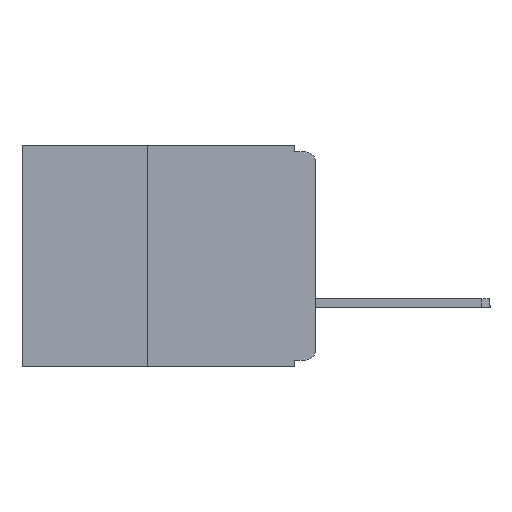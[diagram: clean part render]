
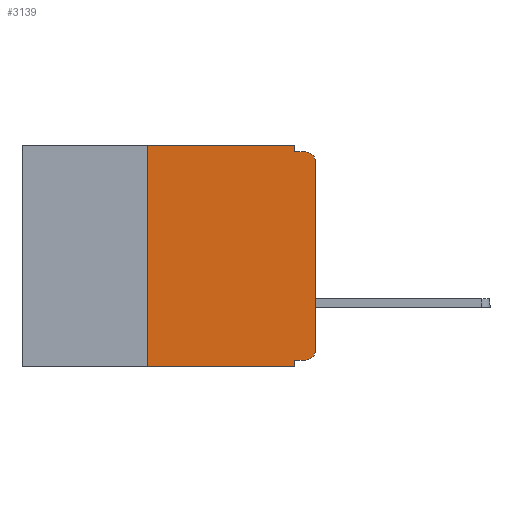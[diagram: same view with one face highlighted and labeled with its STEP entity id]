
A CAD part, left-side view. The second image highlights one B-rep face of the part: STEP entity #3139.
In plain terms, the highlighted planar face has unit normal (-1, 0, 0).
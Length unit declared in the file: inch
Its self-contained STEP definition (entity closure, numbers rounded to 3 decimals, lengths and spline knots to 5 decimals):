
#608 = LINE ( 'NONE', #33275, #14119 ) ;
#1898 = CARTESIAN_POINT ( 'NONE',  ( 0., 0.25, -0.33 ) ) ;
#2515 = CARTESIAN_POINT ( 'NONE',  ( 0., 0., 0. ) ) ;
#2566 = CARTESIAN_POINT ( 'NONE',  ( 0., 0.25, 0. ) ) ;
#3139 = ADVANCED_FACE ( 'NONE', ( #21824 ), #23279, .F. ) ;
#3199 = VERTEX_POINT ( 'NONE', #20405 ) ;
#3339 = ORIENTED_EDGE ( 'NONE', *, *, #6237, .F. ) ;
#4560 = LINE ( 'NONE', #33497, #31786 ) ;
#4748 = VERTEX_POINT ( 'NONE', #15041 ) ;
#5008 = CARTESIAN_POINT ( 'NONE',  ( 0., 0.015, -0.01 ) ) ;
#5044 = ORIENTED_EDGE ( 'NONE', *, *, #23647, .F. ) ;
#5058 = EDGE_LOOP ( 'NONE', ( #14298, #30668, #3339, #17620, #5044, #19236, #20870, #14730, #24922, #26579 ) ) ;
#5066 = VERTEX_POINT ( 'NONE', #10063 ) ;
#5344 = VERTEX_POINT ( 'NONE', #5008 ) ;
#5738 = VECTOR ( 'NONE', #20598, 39.37008 ) ;
#6003 = DIRECTION ( 'NONE',  ( -1., 0., 0. ) ) ;
#6237 = EDGE_CURVE ( 'NONE', #25478, #5344, #15923, .T. ) ;
#6511 = VERTEX_POINT ( 'NONE', #30363 ) ;
#6776 = VERTEX_POINT ( 'NONE', #28749 ) ;
#7833 = EDGE_CURVE ( 'NONE', #6776, #23293, #20725, .T. ) ;
#7985 = VECTOR ( 'NONE', #23960, 39.37008 ) ;
#8428 = EDGE_CURVE ( 'NONE', #5066, #16744, #608, .T. ) ;
#8774 = LINE ( 'NONE', #23782, #21980 ) ;
#8851 = LINE ( 'NONE', #25400, #15092 ) ;
#10063 = CARTESIAN_POINT ( 'NONE',  ( 0., 0.031, -0.32 ) ) ;
#10379 = VERTEX_POINT ( 'NONE', #13954 ) ;
#11586 = AXIS2_PLACEMENT_3D ( 'NONE', #22886, #22854, #22810 ) ;
#12396 = DIRECTION ( 'NONE',  ( 0., 0., -1. ) ) ;
#12749 = DIRECTION ( 'NONE',  ( 0., 1., 0. ) ) ;
#13954 = CARTESIAN_POINT ( 'NONE',  ( 0., 0.015, -0.32 ) ) ;
#14119 = VECTOR ( 'NONE', #12396, 39.37008 ) ;
#14218 = AXIS2_PLACEMENT_3D ( 'NONE', #21885, #6003, #24488 ) ;
#14298 = ORIENTED_EDGE ( 'NONE', *, *, #17887, .T. ) ;
#14347 = CARTESIAN_POINT ( 'NONE',  ( 0., 0.015, -0.305 ) ) ;
#14730 = ORIENTED_EDGE ( 'NONE', *, *, #8428, .F. ) ;
#15041 = CARTESIAN_POINT ( 'NONE',  ( 0., 0., -0.025 ) ) ;
#15092 = VECTOR ( 'NONE', #28047, 39.37008 ) ;
#15923 = LINE ( 'NONE', #21362, #7985 ) ;
#16331 = EDGE_CURVE ( 'NONE', #10379, #5066, #4560, .T. ) ;
#16744 = VERTEX_POINT ( 'NONE', #22338 ) ;
#16999 = DIRECTION ( 'NONE',  ( 0., 0., -1. ) ) ;
#17432 = VECTOR ( 'NONE', #18570, 39.37008 ) ;
#17620 = ORIENTED_EDGE ( 'NONE', *, *, #28528, .F. ) ;
#17887 = EDGE_CURVE ( 'NONE', #3199, #4748, #23500, .T. ) ;
#18570 = DIRECTION ( 'NONE',  ( 0., 0., 1. ) ) ;
#18691 = DIRECTION ( 'NONE',  ( 0., -1., 0. ) ) ;
#19236 = ORIENTED_EDGE ( 'NONE', *, *, #7833, .F. ) ;
#20405 = CARTESIAN_POINT ( 'NONE',  ( 0., 0., -0.305 ) ) ;
#20598 = DIRECTION ( 'NONE',  ( 0., 0., 1. ) ) ;
#20725 = LINE ( 'NONE', #1898, #5738 ) ;
#20870 = ORIENTED_EDGE ( 'NONE', *, *, #29078, .T. ) ;
#21186 = CIRCLE ( 'NONE', #14218, 0.015 ) ;
#21362 = CARTESIAN_POINT ( 'NONE',  ( 0., 0., -0.01 ) ) ;
#21824 = FACE_OUTER_BOUND ( 'NONE', #5058, .T. ) ;
#21885 = CARTESIAN_POINT ( 'NONE',  ( 0., 0.015, -0.025 ) ) ;
#21980 = VECTOR ( 'NONE', #18691, 39.37008 ) ;
#22338 = CARTESIAN_POINT ( 'NONE',  ( 0., 0.031, -0.33 ) ) ;
#22810 = DIRECTION ( 'NONE',  ( 0., 0., -1. ) ) ;
#22854 = DIRECTION ( 'NONE',  ( 1., 0., 0. ) ) ;
#22886 = CARTESIAN_POINT ( 'NONE',  ( 0., 0.437, 0. ) ) ;
#23279 = PLANE ( 'NONE',  #11586 ) ;
#23293 = VERTEX_POINT ( 'NONE', #2566 ) ;
#23500 = LINE ( 'NONE', #2515, #17432 ) ;
#23647 = EDGE_CURVE ( 'NONE', #23293, #6511, #8851, .T. ) ;
#23782 = CARTESIAN_POINT ( 'NONE',  ( 0., 0.437, -0.33 ) ) ;
#23960 = DIRECTION ( 'NONE',  ( 0., -1., 0. ) ) ;
#24488 = DIRECTION ( 'NONE',  ( 0., 0., -1. ) ) ;
#24922 = ORIENTED_EDGE ( 'NONE', *, *, #16331, .F. ) ;
#25247 = VECTOR ( 'NONE', #31579, 39.37008 ) ;
#25400 = CARTESIAN_POINT ( 'NONE',  ( 0., 0.437, 0. ) ) ;
#25478 = VERTEX_POINT ( 'NONE', #34241 ) ;
#26088 = LINE ( 'NONE', #28975, #25247 ) ;
#26220 = AXIS2_PLACEMENT_3D ( 'NONE', #14347, #32568, #16999 ) ;
#26579 = ORIENTED_EDGE ( 'NONE', *, *, #27469, .T. ) ;
#27469 = EDGE_CURVE ( 'NONE', #10379, #3199, #31872, .T. ) ;
#28047 = DIRECTION ( 'NONE',  ( 0., -1., 0. ) ) ;
#28528 = EDGE_CURVE ( 'NONE', #6511, #25478, #26088, .T. ) ;
#28682 = EDGE_CURVE ( 'NONE', #4748, #5344, #21186, .T. ) ;
#28749 = CARTESIAN_POINT ( 'NONE',  ( 0., 0.25, -0.33 ) ) ;
#28975 = CARTESIAN_POINT ( 'NONE',  ( 0., 0.031, 0. ) ) ;
#29078 = EDGE_CURVE ( 'NONE', #6776, #16744, #8774, .T. ) ;
#30363 = CARTESIAN_POINT ( 'NONE',  ( 0., 0.031, 0. ) ) ;
#30668 = ORIENTED_EDGE ( 'NONE', *, *, #28682, .T. ) ;
#31579 = DIRECTION ( 'NONE',  ( 0., 0., -1. ) ) ;
#31786 = VECTOR ( 'NONE', #12749, 39.37008 ) ;
#31872 = CIRCLE ( 'NONE', #26220, 0.015 ) ;
#32568 = DIRECTION ( 'NONE',  ( -1., 0., 0. ) ) ;
#33275 = CARTESIAN_POINT ( 'NONE',  ( 0., 0.031, -0.33 ) ) ;
#33497 = CARTESIAN_POINT ( 'NONE',  ( 0., 0., -0.32 ) ) ;
#34241 = CARTESIAN_POINT ( 'NONE',  ( 0., 0.031, -0.01 ) ) ;
